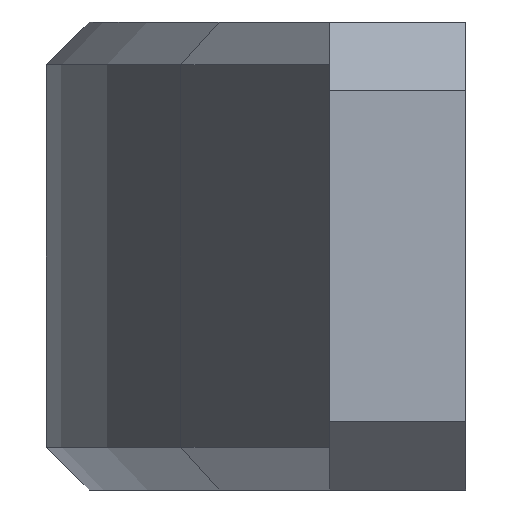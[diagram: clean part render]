
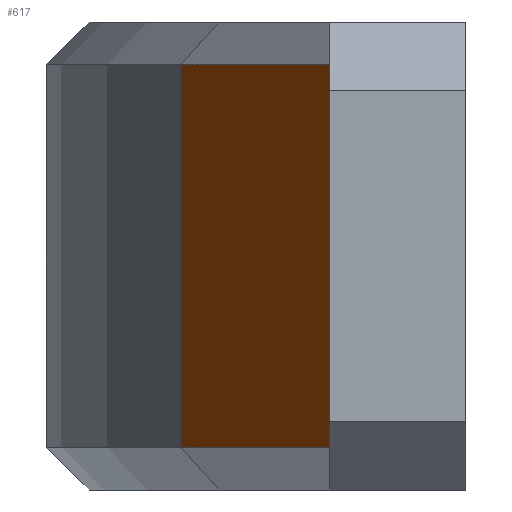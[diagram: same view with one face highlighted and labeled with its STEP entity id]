
A CAD part, left-side view. The second image highlights one B-rep face of the part: STEP entity #617.
In plain terms, the highlighted planar face has unit normal (-0.459, 0.888, 0).
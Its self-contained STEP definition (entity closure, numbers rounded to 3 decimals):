
#19 = LINE ( 'NONE', #773, #402 ) ;
#38 = ORIENTED_EDGE ( 'NONE', *, *, #663, .T. ) ;
#46 = VECTOR ( 'NONE', #700, 1000. ) ;
#84 = EDGE_CURVE ( 'NONE', #822, #321, #19, .T. ) ;
#96 = VERTEX_POINT ( 'NONE', #434 ) ;
#112 = CARTESIAN_POINT ( 'NONE',  ( -12.932, 3.472, 4.461 ) ) ;
#130 = ORIENTED_EDGE ( 'NONE', *, *, #768, .T. ) ;
#146 = AXIS2_PLACEMENT_3D ( 'NONE', #834, #615, #910 ) ;
#179 = VECTOR ( 'NONE', #421, 1000. ) ;
#253 = CARTESIAN_POINT ( 'NONE',  ( -19.653, 0., -4.461 ) ) ;
#279 = DIRECTION ( 'NONE',  ( -0.888, -0.459, 0. ) ) ;
#300 = CARTESIAN_POINT ( 'NONE',  ( -12.932, 3.472, -4.461 ) ) ;
#321 = VERTEX_POINT ( 'NONE', #300 ) ;
#344 = LINE ( 'NONE', #696, #592 ) ;
#363 = LINE ( 'NONE', #858, #179 ) ;
#369 = CARTESIAN_POINT ( 'NONE',  ( -19.653, 0., -5.461 ) ) ;
#402 = VECTOR ( 'NONE', #425, 1000. ) ;
#421 = DIRECTION ( 'NONE',  ( 0.888, 0.459, 0. ) ) ;
#425 = DIRECTION ( 'NONE',  ( 0., 0., -1. ) ) ;
#434 = CARTESIAN_POINT ( 'NONE',  ( -19.653, 0., 4.461 ) ) ;
#546 = VERTEX_POINT ( 'NONE', #253 ) ;
#560 = ORIENTED_EDGE ( 'NONE', *, *, #84, .T. ) ;
#592 = VECTOR ( 'NONE', #279, 1000. ) ;
#615 = DIRECTION ( 'NONE',  ( -0.459, 0.888, 0. ) ) ;
#617 = ADVANCED_FACE ( 'NONE', ( #842 ), #755, .T. ) ;
#663 = EDGE_CURVE ( 'NONE', #321, #546, #344, .T. ) ;
#693 = ORIENTED_EDGE ( 'NONE', *, *, #732, .T. ) ;
#696 = CARTESIAN_POINT ( 'NONE',  ( -19.653, 0., -4.461 ) ) ;
#700 = DIRECTION ( 'NONE',  ( 0., 0., 1. ) ) ;
#732 = EDGE_CURVE ( 'NONE', #546, #96, #903, .T. ) ;
#755 = PLANE ( 'NONE',  #146 ) ;
#768 = EDGE_CURVE ( 'NONE', #96, #822, #363, .T. ) ;
#773 = CARTESIAN_POINT ( 'NONE',  ( -12.932, 3.472, 45.967 ) ) ;
#812 = EDGE_LOOP ( 'NONE', ( #693, #130, #560, #38 ) ) ;
#822 = VERTEX_POINT ( 'NONE', #112 ) ;
#834 = CARTESIAN_POINT ( 'NONE',  ( -4.14, 8.014, 45.967 ) ) ;
#842 = FACE_OUTER_BOUND ( 'NONE', #812, .T. ) ;
#858 = CARTESIAN_POINT ( 'NONE',  ( -4.14, 8.014, 4.461 ) ) ;
#903 = LINE ( 'NONE', #369, #46 ) ;
#910 = DIRECTION ( 'NONE',  ( -0.888, -0.459, 0. ) ) ;
